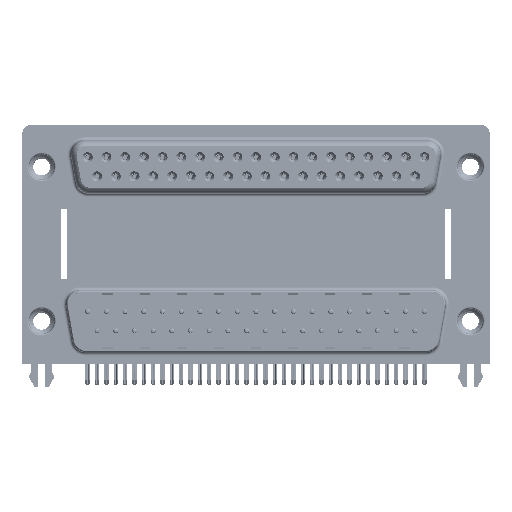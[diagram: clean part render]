
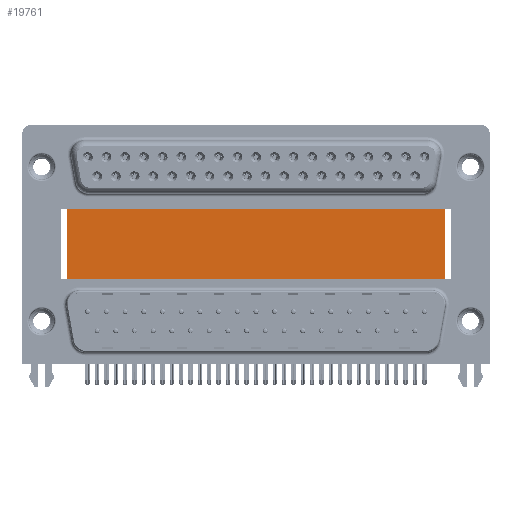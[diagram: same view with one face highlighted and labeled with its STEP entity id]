
A CAD part, top view. The second image highlights one B-rep face of the part: STEP entity #19761.
In plain terms, the highlighted planar face has unit normal (0, 0, 1).
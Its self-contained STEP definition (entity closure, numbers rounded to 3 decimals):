
#2074 = VECTOR ( 'NONE', #42427, 1000. ) ;
#2791 = DIRECTION ( 'NONE',  ( -1., 0., 0. ) ) ;
#6903 = LINE ( 'NONE', #28395, #29097 ) ;
#9465 = PLANE ( 'NONE',  #61688 ) ;
#11128 = VERTEX_POINT ( 'NONE', #68290 ) ;
#11485 = VERTEX_POINT ( 'NONE', #56206 ) ;
#12643 = EDGE_CURVE ( 'NONE', #11485, #11128, #18237, .T. ) ;
#13307 = DIRECTION ( 'NONE',  ( 0., -1., 0. ) ) ;
#14357 = VERTEX_POINT ( 'NONE', #34250 ) ;
#15648 = EDGE_LOOP ( 'NONE', ( #65558, #36073, #26474, #54748 ) ) ;
#16343 = LINE ( 'NONE', #64245, #2074 ) ;
#18237 = LINE ( 'NONE', #18572, #33883 ) ;
#18572 = CARTESIAN_POINT ( 'NONE',  ( 59.71, 16.585, -12. ) ) ;
#19345 = DIRECTION ( 'NONE',  ( 0., 0., -1. ) ) ;
#19761 = ADVANCED_FACE ( 'NONE', ( #68605 ), #9465, .F. ) ;
#22513 = EDGE_CURVE ( 'NONE', #33601, #14357, #6903, .T. ) ;
#22802 = EDGE_CURVE ( 'NONE', #33601, #11485, #16343, .T. ) ;
#26474 = ORIENTED_EDGE ( 'NONE', *, *, #22802, .F. ) ;
#28395 = CARTESIAN_POINT ( 'NONE',  ( 3.79, 16.585, -12. ) ) ;
#29097 = VECTOR ( 'NONE', #49854, 1000. ) ;
#30599 = CARTESIAN_POINT ( 'NONE',  ( 3.79, 16.585, -12. ) ) ;
#33601 = VERTEX_POINT ( 'NONE', #56911 ) ;
#33883 = VECTOR ( 'NONE', #13307, 1000. ) ;
#34250 = CARTESIAN_POINT ( 'NONE',  ( 3.79, -3.735, -12. ) ) ;
#36073 = ORIENTED_EDGE ( 'NONE', *, *, #12643, .F. ) ;
#36422 = EDGE_CURVE ( 'NONE', #14357, #11128, #65888, .T. ) ;
#37700 = VECTOR ( 'NONE', #45109, 1000. ) ;
#42427 = DIRECTION ( 'NONE',  ( 1., 0., 0. ) ) ;
#45109 = DIRECTION ( 'NONE',  ( 1., 0., 0. ) ) ;
#49854 = DIRECTION ( 'NONE',  ( 0., -1., 0. ) ) ;
#54748 = ORIENTED_EDGE ( 'NONE', *, *, #22513, .T. ) ;
#56206 = CARTESIAN_POINT ( 'NONE',  ( 59.71, 16.585, -12. ) ) ;
#56911 = CARTESIAN_POINT ( 'NONE',  ( 3.79, 16.585, -12. ) ) ;
#60616 = CARTESIAN_POINT ( 'NONE',  ( 3.79, -3.735, -12. ) ) ;
#61688 = AXIS2_PLACEMENT_3D ( 'NONE', #30599, #19345, #2791 ) ;
#64245 = CARTESIAN_POINT ( 'NONE',  ( 3.79, 16.585, -12. ) ) ;
#65558 = ORIENTED_EDGE ( 'NONE', *, *, #36422, .T. ) ;
#65888 = LINE ( 'NONE', #60616, #37700 ) ;
#68290 = CARTESIAN_POINT ( 'NONE',  ( 59.71, -3.735, -12. ) ) ;
#68605 = FACE_OUTER_BOUND ( 'NONE', #15648, .T. ) ;
